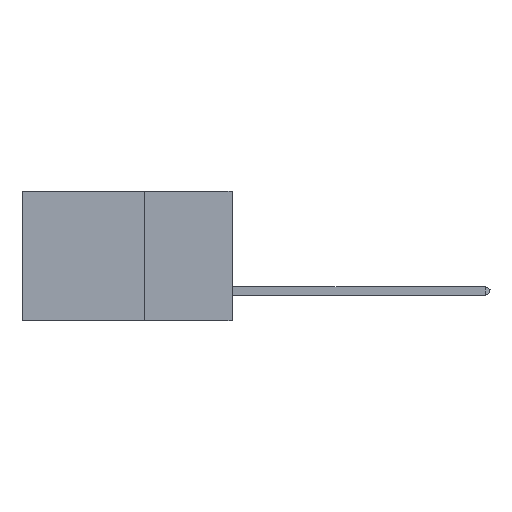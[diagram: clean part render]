
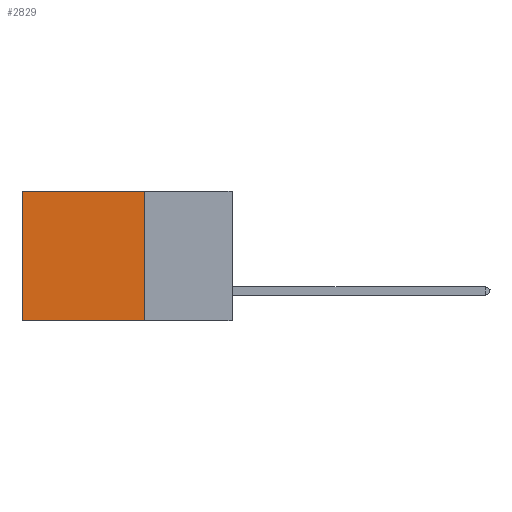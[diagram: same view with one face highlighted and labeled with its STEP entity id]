
A CAD part, left-side view. The second image highlights one B-rep face of the part: STEP entity #2829.
In plain terms, the highlighted planar face has unit normal (-1, 0, 0).
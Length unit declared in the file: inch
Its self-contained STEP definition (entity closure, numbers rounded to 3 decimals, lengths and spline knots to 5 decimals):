
#2829 = ADVANCED_FACE ( 'NONE', ( #12389 ), #30000, .F. ) ;
#5550 = EDGE_CURVE ( 'NONE', #7451, #9997, #11591, .T. ) ;
#6088 = LINE ( 'NONE', #20416, #14690 ) ;
#7451 = VERTEX_POINT ( 'NONE', #44639 ) ;
#7948 = ORIENTED_EDGE ( 'NONE', *, *, #40630, .T. ) ;
#8030 = DIRECTION ( 'NONE',  ( 1., 0., 0. ) ) ;
#8366 = VECTOR ( 'NONE', #37314, 39.37008 ) ;
#8714 = ORIENTED_EDGE ( 'NONE', *, *, #25419, .F. ) ;
#8896 = AXIS2_PLACEMENT_3D ( 'NONE', #37834, #8030, #34158 ) ;
#9997 = VERTEX_POINT ( 'NONE', #31173 ) ;
#10621 = VERTEX_POINT ( 'NONE', #11415 ) ;
#11415 = CARTESIAN_POINT ( 'NONE',  ( 0.2875, 0.25, 0. ) ) ;
#11459 = DIRECTION ( 'NONE',  ( 0., 0., -1. ) ) ;
#11591 = LINE ( 'NONE', #31769, #29425 ) ;
#12038 = EDGE_CURVE ( 'NONE', #10621, #47011, #6088, .T. ) ;
#12389 = FACE_OUTER_BOUND ( 'NONE', #20397, .T. ) ;
#14690 = VECTOR ( 'NONE', #11459, 39.37008 ) ;
#16453 = CARTESIAN_POINT ( 'NONE',  ( 0.2875, 0.25, -0.37 ) ) ;
#20397 = EDGE_LOOP ( 'NONE', ( #28351, #8714, #28173, #7948 ) ) ;
#20416 = CARTESIAN_POINT ( 'NONE',  ( 0.2875, 0.25, 0. ) ) ;
#21076 = LINE ( 'NONE', #47500, #29129 ) ;
#25419 = EDGE_CURVE ( 'NONE', #47011, #9997, #21076, .T. ) ;
#28173 = ORIENTED_EDGE ( 'NONE', *, *, #12038, .F. ) ;
#28351 = ORIENTED_EDGE ( 'NONE', *, *, #5550, .T. ) ;
#29129 = VECTOR ( 'NONE', #43930, 39.37008 ) ;
#29425 = VECTOR ( 'NONE', #47039, 39.37008 ) ;
#30000 = PLANE ( 'NONE',  #8896 ) ;
#31173 = CARTESIAN_POINT ( 'NONE',  ( 0.2875, 0.6, -0.37 ) ) ;
#31769 = CARTESIAN_POINT ( 'NONE',  ( 0.2875, 0.6, 0. ) ) ;
#32887 = CARTESIAN_POINT ( 'NONE',  ( 0.2875, 0.25, 0. ) ) ;
#34158 = DIRECTION ( 'NONE',  ( 0., 0., -1. ) ) ;
#37314 = DIRECTION ( 'NONE',  ( 0., 1., 0. ) ) ;
#37834 = CARTESIAN_POINT ( 'NONE',  ( 0.2875, 0.25, 0. ) ) ;
#40630 = EDGE_CURVE ( 'NONE', #10621, #7451, #41605, .T. ) ;
#41605 = LINE ( 'NONE', #32887, #8366 ) ;
#43930 = DIRECTION ( 'NONE',  ( 0., 1., 0. ) ) ;
#44639 = CARTESIAN_POINT ( 'NONE',  ( 0.2875, 0.6, 0. ) ) ;
#47011 = VERTEX_POINT ( 'NONE', #16453 ) ;
#47039 = DIRECTION ( 'NONE',  ( 0., 0., -1. ) ) ;
#47500 = CARTESIAN_POINT ( 'NONE',  ( 0.2875, 0.25, -0.37 ) ) ;
